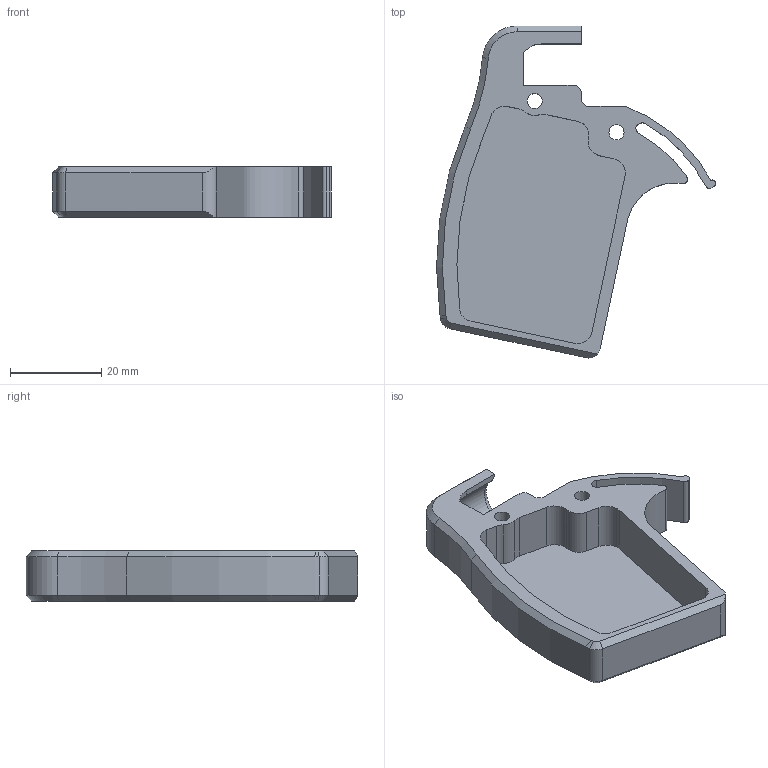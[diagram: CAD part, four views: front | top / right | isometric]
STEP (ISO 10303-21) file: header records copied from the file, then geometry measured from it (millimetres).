
FILE_DESCRIPTION(/* description */ ('STEP AP242','CAx-IF Rec.Pracs.---Representation and Presentation of Product Manufacturing Information (PMI)---4.0---2014-10-13','CAx-IF Rec.Pracs.---3D Tessellated Geometry---0.4---2014-09-14','2;1'),/* implementation_level */ '2;1');
FILE_NAME(/* name */ '61eb2cd132397a7ea2097ddd',/* time_stamp */ '2022-01-21T21:59:45+00:00',/* author */ (''),/* organization */ (''),/* preprocessor_version */ 'ST-DEVELOPER v18.101',/* originating_system */ ' ',/* authorisation */ ' ');
FILE_SCHEMA (('AP242_MANAGED_MODEL_BASED_3D_ENGINEERING_MIM_LF { 1 0 10303 442 1 1 4 }'));
Length unit declared in the file: metre
Products named in the file (1): UFA compliant grip spacer
Bounding box: 61.01 x 72.61 x 11 mm (x, y, z)
Volume: 10912.3 mm3; surface area: 9558.9 mm2
Topology: 1 solids, 1 shells, 68 faces, 185 edges, 120 vertices
Faces by surface type: cylinder 32, plane 25, cone 10, torus 1
Full cylindrical faces by diameter (mm): 3.302 x2
Entity records: 2199 total; most frequent: CARTESIAN_POINT 399, DIRECTION 392, ORIENTED_EDGE 366, EDGE_CURVE 183, AXIS2_PLACEMENT_3D 148, VERTEX_POINT 120, LINE 96, VECTOR 96
